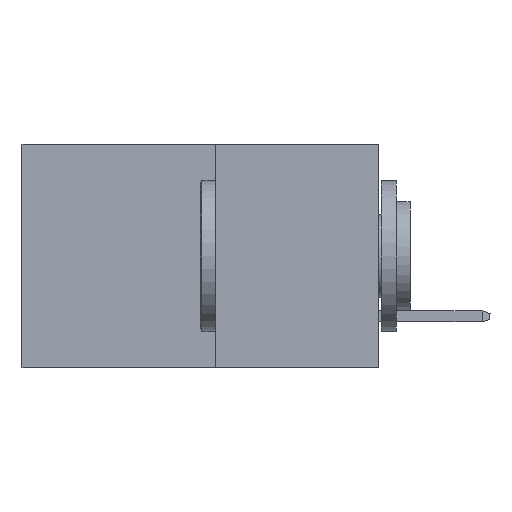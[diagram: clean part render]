
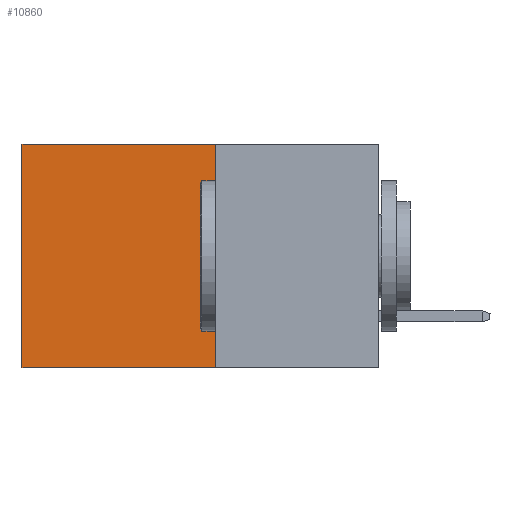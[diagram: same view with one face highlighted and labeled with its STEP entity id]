
A CAD part, left-side view. The second image highlights one B-rep face of the part: STEP entity #10860.
In plain terms, the highlighted planar face has unit normal (-1, 0, 0).
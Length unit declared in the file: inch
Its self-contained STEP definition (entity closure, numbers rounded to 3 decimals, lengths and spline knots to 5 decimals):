
#228 = CARTESIAN_POINT ( 'NONE',  ( 0.277, 0.27, 0. ) ) ;
#565 = LINE ( 'NONE', #2551, #5743 ) ;
#981 = VERTEX_POINT ( 'NONE', #2213 ) ;
#1374 = CARTESIAN_POINT ( 'NONE',  ( 0.277, 0.27, 0. ) ) ;
#2213 = CARTESIAN_POINT ( 'NONE',  ( 0.277, 0.27, -0.37 ) ) ;
#2551 = CARTESIAN_POINT ( 'NONE',  ( 0.277, 0.59, -0.37 ) ) ;
#2575 = LINE ( 'NONE', #228, #12188 ) ;
#3666 = ORIENTED_EDGE ( 'NONE', *, *, #12163, .F. ) ;
#5508 = CARTESIAN_POINT ( 'NONE',  ( 0.277, 0.59, 0. ) ) ;
#5743 = VECTOR ( 'NONE', #11429, 39.37008 ) ;
#5971 = ORIENTED_EDGE ( 'NONE', *, *, #11616, .T. ) ;
#6057 = DIRECTION ( 'NONE',  ( 0., 1., 0. ) ) ;
#6610 = CARTESIAN_POINT ( 'NONE',  ( 0.277, 0.27, -0.37 ) ) ;
#6626 = DIRECTION ( 'NONE',  ( 0., 1., 0. ) ) ;
#6765 = CARTESIAN_POINT ( 'NONE',  ( 0.277, 0.59, -0.37 ) ) ;
#7478 = DIRECTION ( 'NONE',  ( 0., 0., -1. ) ) ;
#7770 = DIRECTION ( 'NONE',  ( 1., 0., 0. ) ) ;
#8726 = EDGE_CURVE ( 'NONE', #981, #9605, #11773, .T. ) ;
#9605 = VERTEX_POINT ( 'NONE', #6765 ) ;
#10077 = VERTEX_POINT ( 'NONE', #5508 ) ;
#10364 = EDGE_LOOP ( 'NONE', ( #5971, #10681, #3666, #11571 ) ) ;
#10440 = EDGE_CURVE ( 'NONE', #10563, #10077, #2575, .T. ) ;
#10444 = AXIS2_PLACEMENT_3D ( 'NONE', #10726, #7770, #12603 ) ;
#10563 = VERTEX_POINT ( 'NONE', #1374 ) ;
#10681 = ORIENTED_EDGE ( 'NONE', *, *, #8726, .F. ) ;
#10726 = CARTESIAN_POINT ( 'NONE',  ( 0.277, 0.27, -0.37 ) ) ;
#10860 = ADVANCED_FACE ( 'NONE', ( #12367 ), #11673, .F. ) ;
#10866 = VECTOR ( 'NONE', #7478, 39.37008 ) ;
#11166 = LINE ( 'NONE', #12307, #10866 ) ;
#11429 = DIRECTION ( 'NONE',  ( 0., 0., -1. ) ) ;
#11484 = VECTOR ( 'NONE', #6626, 39.37008 ) ;
#11571 = ORIENTED_EDGE ( 'NONE', *, *, #10440, .T. ) ;
#11616 = EDGE_CURVE ( 'NONE', #10077, #9605, #565, .T. ) ;
#11673 = PLANE ( 'NONE',  #10444 ) ;
#11773 = LINE ( 'NONE', #6610, #11484 ) ;
#12163 = EDGE_CURVE ( 'NONE', #10563, #981, #11166, .T. ) ;
#12188 = VECTOR ( 'NONE', #6057, 39.37008 ) ;
#12307 = CARTESIAN_POINT ( 'NONE',  ( 0.277, 0.27, -0.37 ) ) ;
#12367 = FACE_OUTER_BOUND ( 'NONE', #10364, .T. ) ;
#12603 = DIRECTION ( 'NONE',  ( 0., 0., -1. ) ) ;
